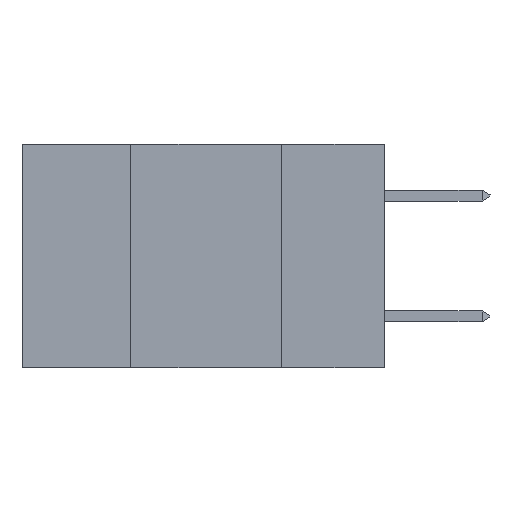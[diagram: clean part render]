
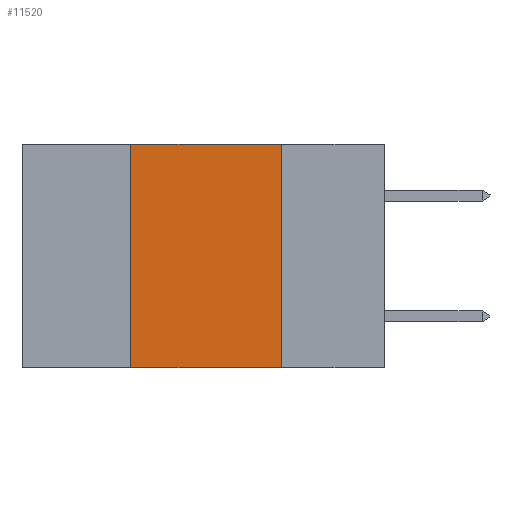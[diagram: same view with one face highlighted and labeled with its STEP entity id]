
A CAD part, left-side view. The second image highlights one B-rep face of the part: STEP entity #11520.
In plain terms, the highlighted planar face has unit normal (-1, 0, 0).
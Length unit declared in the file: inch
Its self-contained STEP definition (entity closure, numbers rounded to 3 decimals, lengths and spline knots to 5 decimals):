
#146 = PLANE ( 'NONE',  #4884 ) ;
#692 = EDGE_LOOP ( 'NONE', ( #1697, #7277, #13182, #11269 ) ) ;
#938 = CARTESIAN_POINT ( 'NONE',  ( 0., 0.42, -0.37 ) ) ;
#1038 = DIRECTION ( 'NONE',  ( 0., 0., 1. ) ) ;
#1697 = ORIENTED_EDGE ( 'NONE', *, *, #13761, .F. ) ;
#2649 = VERTEX_POINT ( 'NONE', #11054 ) ;
#3094 = DIRECTION ( 'NONE',  ( 1., 0., 0. ) ) ;
#4221 = VECTOR ( 'NONE', #6386, 39.37008 ) ;
#4884 = AXIS2_PLACEMENT_3D ( 'NONE', #9243, #3094, #10647 ) ;
#4945 = LINE ( 'NONE', #11466, #6831 ) ;
#5705 = VERTEX_POINT ( 'NONE', #11426 ) ;
#6015 = LINE ( 'NONE', #12931, #10955 ) ;
#6386 = DIRECTION ( 'NONE',  ( 0., -1., 0. ) ) ;
#6534 = LINE ( 'NONE', #9580, #13565 ) ;
#6831 = VECTOR ( 'NONE', #13660, 39.37008 ) ;
#7064 = EDGE_CURVE ( 'NONE', #5705, #12621, #6015, .T. ) ;
#7277 = ORIENTED_EDGE ( 'NONE', *, *, #7064, .F. ) ;
#7371 = VERTEX_POINT ( 'NONE', #938 ) ;
#8576 = DIRECTION ( 'NONE',  ( 0., -1., 0. ) ) ;
#8925 = CARTESIAN_POINT ( 'NONE',  ( 0., 0.17, 0. ) ) ;
#9243 = CARTESIAN_POINT ( 'NONE',  ( 0., 0.6, 0. ) ) ;
#9580 = CARTESIAN_POINT ( 'NONE',  ( 0., 0.42, 0. ) ) ;
#9648 = EDGE_CURVE ( 'NONE', #7371, #2649, #12782, .T. ) ;
#10647 = DIRECTION ( 'NONE',  ( 0., 0., -1. ) ) ;
#10955 = VECTOR ( 'NONE', #8576, 39.37008 ) ;
#11054 = CARTESIAN_POINT ( 'NONE',  ( 0., 0.17, -0.37 ) ) ;
#11269 = ORIENTED_EDGE ( 'NONE', *, *, #9648, .T. ) ;
#11330 = FACE_OUTER_BOUND ( 'NONE', #692, .T. ) ;
#11426 = CARTESIAN_POINT ( 'NONE',  ( 0., 0.42, 0. ) ) ;
#11466 = CARTESIAN_POINT ( 'NONE',  ( 0., 0.17, 0. ) ) ;
#11520 = ADVANCED_FACE ( 'NONE', ( #11330 ), #146, .F. ) ;
#12069 = EDGE_CURVE ( 'NONE', #7371, #5705, #6534, .T. ) ;
#12621 = VERTEX_POINT ( 'NONE', #8925 ) ;
#12782 = LINE ( 'NONE', #14108, #4221 ) ;
#12931 = CARTESIAN_POINT ( 'NONE',  ( 0., 0.6, 0. ) ) ;
#13182 = ORIENTED_EDGE ( 'NONE', *, *, #12069, .F. ) ;
#13565 = VECTOR ( 'NONE', #1038, 39.37008 ) ;
#13660 = DIRECTION ( 'NONE',  ( 0., 0., -1. ) ) ;
#13761 = EDGE_CURVE ( 'NONE', #12621, #2649, #4945, .T. ) ;
#14108 = CARTESIAN_POINT ( 'NONE',  ( 0., 0.6, -0.37 ) ) ;
